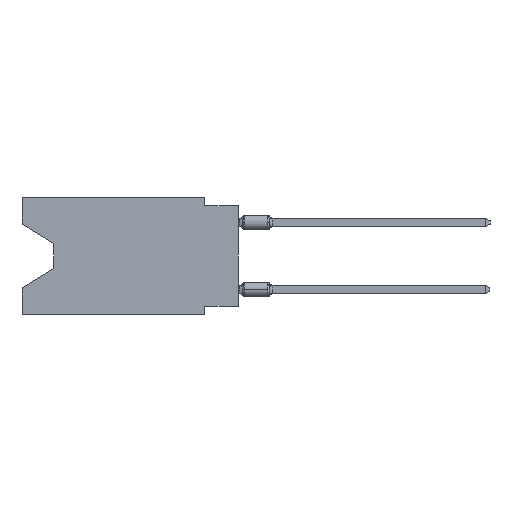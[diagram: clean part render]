
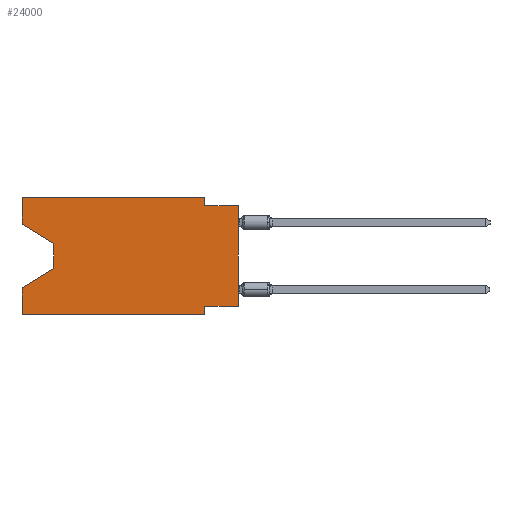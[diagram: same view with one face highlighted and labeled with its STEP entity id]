
A CAD part, left-side view. The second image highlights one B-rep face of the part: STEP entity #24000.
In plain terms, the highlighted planar face has unit normal (-1, 0, 0).
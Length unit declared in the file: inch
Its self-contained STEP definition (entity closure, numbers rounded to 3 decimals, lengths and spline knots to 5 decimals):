
#133 = ORIENTED_EDGE ( 'NONE', *, *, #9708, .T. ) ;
#196 = LINE ( 'NONE', #17142, #2451 ) ;
#523 = DIRECTION ( 'NONE',  ( 0., 0., 1. ) ) ;
#643 = CARTESIAN_POINT ( 'NONE',  ( 0., 0.645, -0.08025 ) ) ;
#866 = DIRECTION ( 'NONE',  ( 1., 0., 0. ) ) ;
#1300 = VECTOR ( 'NONE', #20245, 39.37008 ) ;
#1861 = CARTESIAN_POINT ( 'NONE',  ( 0., 0.1, -0.35 ) ) ;
#2139 = VERTEX_POINT ( 'NONE', #3792 ) ;
#2285 = EDGE_LOOP ( 'NONE', ( #11256, #24884, #13377, #7681, #4450, #16018, #13224, #133, #10269, #15911, #14717, #17010 ) ) ;
#2354 = AXIS2_PLACEMENT_3D ( 'NONE', #22088, #866, #9616 ) ;
#2451 = VECTOR ( 'NONE', #17392, 39.37008 ) ;
#2619 = LINE ( 'NONE', #17330, #3878 ) ;
#3013 = EDGE_CURVE ( 'NONE', #27154, #16449, #6048, .T. ) ;
#3116 = CARTESIAN_POINT ( 'NONE',  ( 0., 0.645, -0.35 ) ) ;
#3792 = CARTESIAN_POINT ( 'NONE',  ( 0., 0.1, 0. ) ) ;
#3878 = VECTOR ( 'NONE', #9292, 39.37008 ) ;
#4287 = CARTESIAN_POINT ( 'NONE',  ( 0., 0.55, -0.138 ) ) ;
#4450 = ORIENTED_EDGE ( 'NONE', *, *, #8071, .T. ) ;
#5945 = EDGE_CURVE ( 'NONE', #15069, #25963, #10961, .T. ) ;
#5965 = VECTOR ( 'NONE', #18490, 39.37008 ) ;
#5994 = LINE ( 'NONE', #14456, #24527 ) ;
#6048 = LINE ( 'NONE', #1861, #23656 ) ;
#6979 = VERTEX_POINT ( 'NONE', #3116 ) ;
#7681 = ORIENTED_EDGE ( 'NONE', *, *, #21875, .F. ) ;
#7977 = CARTESIAN_POINT ( 'NONE',  ( 0., 0.55, -0.212 ) ) ;
#8071 = EDGE_CURVE ( 'NONE', #6979, #16449, #14860, .T. ) ;
#8130 = CARTESIAN_POINT ( 'NONE',  ( 0., 0.645, 0. ) ) ;
#8455 = LINE ( 'NONE', #643, #25066 ) ;
#8577 = LINE ( 'NONE', #21758, #26354 ) ;
#9192 = CARTESIAN_POINT ( 'NONE',  ( 0., 0.645, -0.08025 ) ) ;
#9292 = DIRECTION ( 'NONE',  ( 0., 1., 0. ) ) ;
#9294 = LINE ( 'NONE', #23978, #1300 ) ;
#9616 = DIRECTION ( 'NONE',  ( 0., 0., -1. ) ) ;
#9708 = EDGE_CURVE ( 'NONE', #19709, #25963, #8577, .T. ) ;
#9940 = VECTOR ( 'NONE', #14498, 39.37008 ) ;
#10269 = ORIENTED_EDGE ( 'NONE', *, *, #5945, .F. ) ;
#10618 = CARTESIAN_POINT ( 'NONE',  ( 0., 0.1, -0.325 ) ) ;
#10961 = LINE ( 'NONE', #27358, #20156 ) ;
#11256 = ORIENTED_EDGE ( 'NONE', *, *, #14147, .T. ) ;
#12795 = CARTESIAN_POINT ( 'NONE',  ( 0., 0.645, -0.35 ) ) ;
#13035 = CARTESIAN_POINT ( 'NONE',  ( 0., 0.645, 0. ) ) ;
#13215 = EDGE_CURVE ( 'NONE', #27005, #25226, #26986, .T. ) ;
#13224 = ORIENTED_EDGE ( 'NONE', *, *, #15391, .F. ) ;
#13377 = ORIENTED_EDGE ( 'NONE', *, *, #13215, .T. ) ;
#13456 = EDGE_CURVE ( 'NONE', #2139, #15069, #24863, .T. ) ;
#13583 = CARTESIAN_POINT ( 'NONE',  ( 0., 0., -0.025 ) ) ;
#14147 = EDGE_CURVE ( 'NONE', #17454, #25781, #8455, .T. ) ;
#14178 = DIRECTION ( 'NONE',  ( 0., 0., 1. ) ) ;
#14354 = CARTESIAN_POINT ( 'NONE',  ( 0., 0., -0.325 ) ) ;
#14456 = CARTESIAN_POINT ( 'NONE',  ( 0., 0.645, 0. ) ) ;
#14498 = DIRECTION ( 'NONE',  ( 0., 0.855, -0.519 ) ) ;
#14533 = EDGE_CURVE ( 'NONE', #27094, #2139, #196, .T. ) ;
#14717 = ORIENTED_EDGE ( 'NONE', *, *, #14533, .F. ) ;
#14830 = DIRECTION ( 'NONE',  ( 0., -0.855, -0.519 ) ) ;
#14835 = CARTESIAN_POINT ( 'NONE',  ( 0., 0.1, -0.35 ) ) ;
#14860 = LINE ( 'NONE', #12795, #22420 ) ;
#15069 = VERTEX_POINT ( 'NONE', #15983 ) ;
#15391 = EDGE_CURVE ( 'NONE', #19709, #27154, #2619, .T. ) ;
#15865 = PLANE ( 'NONE',  #2354 ) ;
#15911 = ORIENTED_EDGE ( 'NONE', *, *, #13456, .F. ) ;
#15983 = CARTESIAN_POINT ( 'NONE',  ( 0., 0.1, -0.025 ) ) ;
#16018 = ORIENTED_EDGE ( 'NONE', *, *, #3013, .F. ) ;
#16449 = VERTEX_POINT ( 'NONE', #14835 ) ;
#17010 = ORIENTED_EDGE ( 'NONE', *, *, #24235, .F. ) ;
#17081 = DIRECTION ( 'NONE',  ( 0., -1., 0. ) ) ;
#17142 = CARTESIAN_POINT ( 'NONE',  ( 0., 0.645, 0. ) ) ;
#17330 = CARTESIAN_POINT ( 'NONE',  ( 0., 0., -0.325 ) ) ;
#17392 = DIRECTION ( 'NONE',  ( 0., -1., 0. ) ) ;
#17454 = VERTEX_POINT ( 'NONE', #9192 ) ;
#17878 = EDGE_CURVE ( 'NONE', #25781, #27005, #9294, .T. ) ;
#18206 = CARTESIAN_POINT ( 'NONE',  ( 0., 0.645, -0.26975 ) ) ;
#18490 = DIRECTION ( 'NONE',  ( 0., 0., -1. ) ) ;
#19709 = VERTEX_POINT ( 'NONE', #14354 ) ;
#20156 = VECTOR ( 'NONE', #17081, 39.37008 ) ;
#20245 = DIRECTION ( 'NONE',  ( 0., 0., -1. ) ) ;
#20291 = FACE_OUTER_BOUND ( 'NONE', #2285, .T. ) ;
#21091 = LINE ( 'NONE', #13035, #24323 ) ;
#21227 = DIRECTION ( 'NONE',  ( 0., 0., 1. ) ) ;
#21244 = DIRECTION ( 'NONE',  ( 0., -1., 0. ) ) ;
#21344 = CARTESIAN_POINT ( 'NONE',  ( 0., 0.55, -0.212 ) ) ;
#21758 = CARTESIAN_POINT ( 'NONE',  ( 0., 0., 0. ) ) ;
#21875 = EDGE_CURVE ( 'NONE', #6979, #25226, #21091, .T. ) ;
#22088 = CARTESIAN_POINT ( 'NONE',  ( 0., 0.645, 0. ) ) ;
#22420 = VECTOR ( 'NONE', #21244, 39.37008 ) ;
#23088 = DIRECTION ( 'NONE',  ( 0., 0., -1. ) ) ;
#23656 = VECTOR ( 'NONE', #23088, 39.37008 ) ;
#23978 = CARTESIAN_POINT ( 'NONE',  ( 0., 0.55, -0.138 ) ) ;
#24000 = ADVANCED_FACE ( 'NONE', ( #20291 ), #15865, .F. ) ;
#24235 = EDGE_CURVE ( 'NONE', #17454, #27094, #5994, .T. ) ;
#24323 = VECTOR ( 'NONE', #21227, 39.37008 ) ;
#24527 = VECTOR ( 'NONE', #14178, 39.37008 ) ;
#24863 = LINE ( 'NONE', #26952, #5965 ) ;
#24884 = ORIENTED_EDGE ( 'NONE', *, *, #17878, .T. ) ;
#25066 = VECTOR ( 'NONE', #14830, 39.37008 ) ;
#25226 = VERTEX_POINT ( 'NONE', #18206 ) ;
#25781 = VERTEX_POINT ( 'NONE', #4287 ) ;
#25963 = VERTEX_POINT ( 'NONE', #13583 ) ;
#26354 = VECTOR ( 'NONE', #523, 39.37008 ) ;
#26952 = CARTESIAN_POINT ( 'NONE',  ( 0., 0.1, 0. ) ) ;
#26986 = LINE ( 'NONE', #7977, #9940 ) ;
#27005 = VERTEX_POINT ( 'NONE', #21344 ) ;
#27094 = VERTEX_POINT ( 'NONE', #8130 ) ;
#27154 = VERTEX_POINT ( 'NONE', #10618 ) ;
#27358 = CARTESIAN_POINT ( 'NONE',  ( 0., 0., -0.025 ) ) ;
